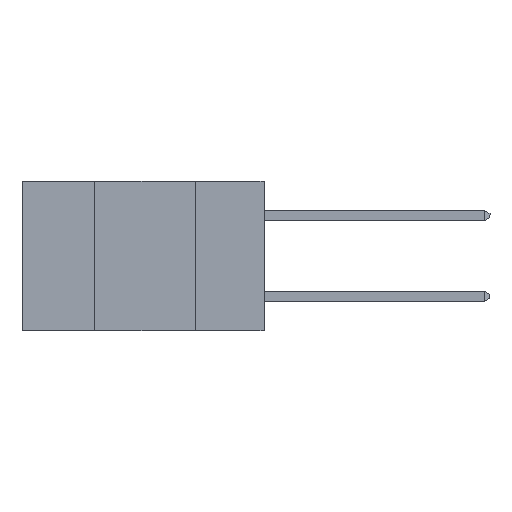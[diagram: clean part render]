
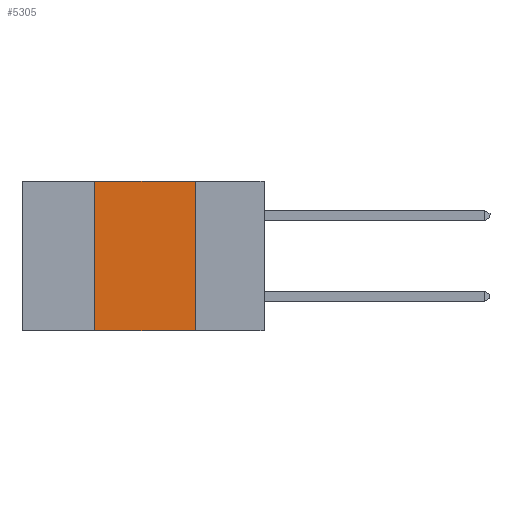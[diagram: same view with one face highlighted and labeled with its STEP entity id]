
A CAD part, left-side view. The second image highlights one B-rep face of the part: STEP entity #5305.
In plain terms, the highlighted planar face has unit normal (-1, 0, 0).
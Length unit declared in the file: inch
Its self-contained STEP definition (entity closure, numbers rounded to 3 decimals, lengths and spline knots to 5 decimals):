
#125 = CARTESIAN_POINT ( 'NONE',  ( 0., 0.6, 0. ) ) ;
#350 = EDGE_LOOP ( 'NONE', ( #8813, #3698, #1147, #6989 ) ) ;
#479 = LINE ( 'NONE', #2663, #5940 ) ;
#932 = VECTOR ( 'NONE', #12710, 39.37008 ) ;
#1053 = DIRECTION ( 'NONE',  ( 0., 0., 1. ) ) ;
#1147 = ORIENTED_EDGE ( 'NONE', *, *, #2637, .F. ) ;
#2381 = EDGE_CURVE ( 'NONE', #8515, #8543, #8177, .T. ) ;
#2637 = EDGE_CURVE ( 'NONE', #8515, #6812, #9524, .T. ) ;
#2663 = CARTESIAN_POINT ( 'NONE',  ( 0., 0.17, 0. ) ) ;
#3253 = EDGE_CURVE ( 'NONE', #5185, #8543, #479, .T. ) ;
#3576 = PLANE ( 'NONE',  #10391 ) ;
#3698 = ORIENTED_EDGE ( 'NONE', *, *, #8008, .F. ) ;
#3800 = LINE ( 'NONE', #8476, #932 ) ;
#3878 = VECTOR ( 'NONE', #1053, 39.37008 ) ;
#5185 = VERTEX_POINT ( 'NONE', #5261 ) ;
#5211 = CARTESIAN_POINT ( 'NONE',  ( 0., 0.42, 0. ) ) ;
#5261 = CARTESIAN_POINT ( 'NONE',  ( 0., 0.17, 0. ) ) ;
#5305 = ADVANCED_FACE ( 'NONE', ( #7002 ), #3576, .F. ) ;
#5431 = VECTOR ( 'NONE', #10099, 39.37008 ) ;
#5940 = VECTOR ( 'NONE', #9335, 39.37008 ) ;
#6550 = DIRECTION ( 'NONE',  ( 0., 0., -1. ) ) ;
#6582 = DIRECTION ( 'NONE',  ( 1., 0., 0. ) ) ;
#6812 = VERTEX_POINT ( 'NONE', #10344 ) ;
#6989 = ORIENTED_EDGE ( 'NONE', *, *, #2381, .T. ) ;
#7002 = FACE_OUTER_BOUND ( 'NONE', #350, .T. ) ;
#8008 = EDGE_CURVE ( 'NONE', #6812, #5185, #3800, .T. ) ;
#8177 = LINE ( 'NONE', #8663, #5431 ) ;
#8476 = CARTESIAN_POINT ( 'NONE',  ( 0., 0.6, 0. ) ) ;
#8515 = VERTEX_POINT ( 'NONE', #8807 ) ;
#8543 = VERTEX_POINT ( 'NONE', #9723 ) ;
#8663 = CARTESIAN_POINT ( 'NONE',  ( 0., 0.6, -0.37 ) ) ;
#8807 = CARTESIAN_POINT ( 'NONE',  ( 0., 0.42, -0.37 ) ) ;
#8813 = ORIENTED_EDGE ( 'NONE', *, *, #3253, .F. ) ;
#9335 = DIRECTION ( 'NONE',  ( 0., 0., -1. ) ) ;
#9524 = LINE ( 'NONE', #5211, #3878 ) ;
#9723 = CARTESIAN_POINT ( 'NONE',  ( 0., 0.17, -0.37 ) ) ;
#10099 = DIRECTION ( 'NONE',  ( 0., -1., 0. ) ) ;
#10344 = CARTESIAN_POINT ( 'NONE',  ( 0., 0.42, 0. ) ) ;
#10391 = AXIS2_PLACEMENT_3D ( 'NONE', #125, #6582, #6550 ) ;
#12710 = DIRECTION ( 'NONE',  ( 0., -1., 0. ) ) ;
